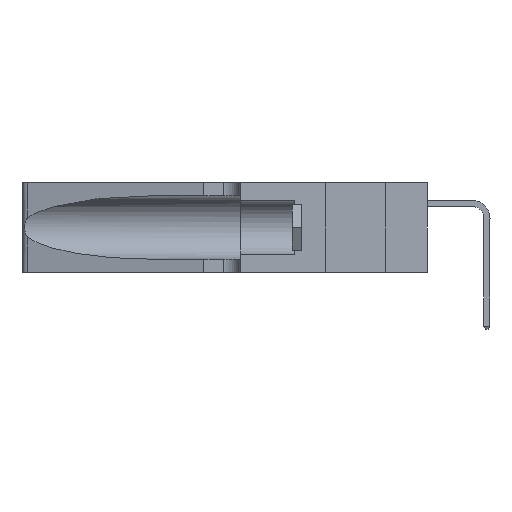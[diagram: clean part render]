
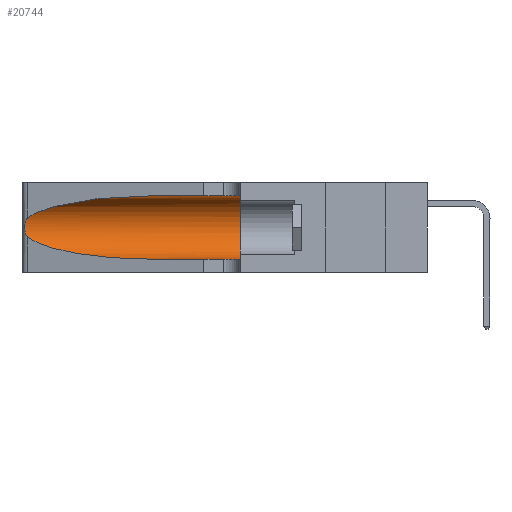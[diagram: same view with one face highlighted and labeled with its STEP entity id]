
A CAD part, left-side view. The second image highlights one B-rep face of the part: STEP entity #20744.
In plain terms, the highlighted cylindrical face has radius 3.308 mm (diameter 6.617 mm), a partial arc.
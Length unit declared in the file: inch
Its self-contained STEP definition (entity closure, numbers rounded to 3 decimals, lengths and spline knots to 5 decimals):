
#2457 = VERTEX_POINT ( 'NONE', #29035 ) ;
#2766 = CARTESIAN_POINT ( 'NONE',  ( 0.18966, 0.96281, 0.31525 ) ) ;
#2930 = CARTESIAN_POINT ( 'NONE',  ( 0.25555, 1.22993, 0.14849 ) ) ;
#2975 = DIRECTION ( 'NONE',  ( 0., 0., 1. ) ) ;
#4434 = CIRCLE ( 'NONE', #12523, 0.13025 ) ;
#4700 = VERTEX_POINT ( 'NONE', #17349 ) ;
#5155 = VERTEX_POINT ( 'NONE', #10146 ) ;
#5742 = VECTOR ( 'NONE', #9427, 39.37008 ) ;
#6196 = ORIENTED_EDGE ( 'NONE', *, *, #11854, .T. ) ;
#7155 = ORIENTED_EDGE ( 'NONE', *, *, #12592, .F. ) ;
#8852 = CARTESIAN_POINT ( 'NONE',  ( 0.25787, 1.23484, 0.2124 ) ) ;
#9427 = DIRECTION ( 'NONE',  ( 0., -1., 0. ) ) ;
#9533 =( BOUNDED_CURVE ( )  B_SPLINE_CURVE ( 3, ( #29793, #2766, #29912, #12100 ),
 .UNSPECIFIED., .F., .F. ) 
 B_SPLINE_CURVE_WITH_KNOTS ( ( 4, 4 ),
 ( 1.5708, 2.84003 ),
 .UNSPECIFIED. ) 
 CURVE ( )  GEOMETRIC_REPRESENTATION_ITEM ( )  RATIONAL_B_SPLINE_CURVE ( ( 1., 0.87, 0.87, 1. ) ) 
 REPRESENTATION_ITEM ( '' )  );
#10146 = CARTESIAN_POINT ( 'NONE',  ( 0.25487, 1.22718, 0.22369 ) ) ;
#10614 = CARTESIAN_POINT ( 'NONE',  ( 0.1305, 0.35, 0.185 ) ) ;
#10757 = ORIENTED_EDGE ( 'NONE', *, *, #21617, .T. ) ;
#11854 = EDGE_CURVE ( 'NONE', #20421, #36447, #29602, .T. ) ;
#11882 = CARTESIAN_POINT ( 'NONE',  ( 0.26018, 1.23835, 0.19895 ) ) ;
#12100 = CARTESIAN_POINT ( 'NONE',  ( 0.25487, 1.22718, 0.22369 ) ) ;
#12523 = AXIS2_PLACEMENT_3D ( 'NONE', #10614, #20919, #2975 ) ;
#12592 = EDGE_CURVE ( 'NONE', #4700, #2457, #34492, .T. ) ;
#13160 = B_SPLINE_CURVE_WITH_KNOTS ( 'NONE', 3,
 ( #38353, #32504, #26718, #8852, #29709, #11882, #32627, #14880, #35553, #17895, #38488, #20868, #2930, #23845 ),
 .UNSPECIFIED., .F., .F.,
 ( 4, 2, 2, 2, 2, 2, 4 ),
 ( 0., 0.00027, 0.00053, 0.00107, 0.0016, 0.00187, 0.00214 ),
 .UNSPECIFIED. ) ;
#14221 = CARTESIAN_POINT ( 'NONE',  ( 0.1305, 0.35, 0.05475 ) ) ;
#14829 = EDGE_CURVE ( 'NONE', #4700, #5155, #9533, .T. ) ;
#14880 = CARTESIAN_POINT ( 'NONE',  ( 0.26075, 1.23896, 0.178 ) ) ;
#15347 = EDGE_CURVE ( 'NONE', #2457, #36447, #4434, .T. ) ;
#15897 = CARTESIAN_POINT ( 'NONE',  ( 0.18966, 0.96281, 0.05475 ) ) ;
#16669 = VERTEX_POINT ( 'NONE', #26943 ) ;
#17170 = AXIS2_PLACEMENT_3D ( 'NONE', #28837, #25985, #20029 ) ;
#17349 = CARTESIAN_POINT ( 'NONE',  ( 0.1305, 0.72297, 0.31525 ) ) ;
#17895 = CARTESIAN_POINT ( 'NONE',  ( 0.25856, 1.23593, 0.16098 ) ) ;
#18598 = CYLINDRICAL_SURFACE ( 'NONE', #17170, 0.13025 ) ;
#18799 = CARTESIAN_POINT ( 'NONE',  ( 0.1305, 1.61858, 0.31525 ) ) ;
#19523 = FACE_OUTER_BOUND ( 'NONE', #21586, .T. ) ;
#20029 = DIRECTION ( 'NONE',  ( 0., 0., -1. ) ) ;
#20421 = VERTEX_POINT ( 'NONE', #33392 ) ;
#20744 = ADVANCED_FACE ( 'NONE', ( #19523 ), #18598, .F. ) ;
#20868 = CARTESIAN_POINT ( 'NONE',  ( 0.25639, 1.23186, 0.15144 ) ) ;
#20919 = DIRECTION ( 'NONE',  ( 0., 1., 0. ) ) ;
#21586 = EDGE_LOOP ( 'NONE', ( #27851, #10757, #31689, #6196, #37943, #7155 ) ) ;
#21617 = EDGE_CURVE ( 'NONE', #5155, #16669, #13160, .T. ) ;
#23845 = CARTESIAN_POINT ( 'NONE',  ( 0.25487, 1.22718, 0.14631 ) ) ;
#24277 = EDGE_CURVE ( 'NONE', #16669, #20421, #29727, .T. ) ;
#24756 = CARTESIAN_POINT ( 'NONE',  ( 0.2373, 1.15595, 0.08982 ) ) ;
#25985 = DIRECTION ( 'NONE',  ( 0., -1., 0. ) ) ;
#26718 = CARTESIAN_POINT ( 'NONE',  ( 0.25639, 1.23184, 0.21858 ) ) ;
#26729 = VECTOR ( 'NONE', #36441, 39.37008 ) ;
#26943 = CARTESIAN_POINT ( 'NONE',  ( 0.25487, 1.22718, 0.14631 ) ) ;
#27733 = CARTESIAN_POINT ( 'NONE',  ( 0.25487, 1.22718, 0.14631 ) ) ;
#27851 = ORIENTED_EDGE ( 'NONE', *, *, #14829, .T. ) ;
#28837 = CARTESIAN_POINT ( 'NONE',  ( 0.1305, 1.61858, 0.185 ) ) ;
#29035 = CARTESIAN_POINT ( 'NONE',  ( 0.1305, 0.35, 0.31525 ) ) ;
#29602 = LINE ( 'NONE', #30263, #5742 ) ;
#29709 = CARTESIAN_POINT ( 'NONE',  ( 0.25854, 1.2359, 0.20912 ) ) ;
#29727 =( BOUNDED_CURVE ( )  B_SPLINE_CURVE ( 3, ( #27733, #24756, #15897, #36566 ),
 .UNSPECIFIED., .F., .F. ) 
 B_SPLINE_CURVE_WITH_KNOTS ( ( 4, 4 ),
 ( 3.44316, 4.71239 ),
 .UNSPECIFIED. ) 
 CURVE ( )  GEOMETRIC_REPRESENTATION_ITEM ( )  RATIONAL_B_SPLINE_CURVE ( ( 1., 0.87, 0.87, 1. ) ) 
 REPRESENTATION_ITEM ( '' )  );
#29793 = CARTESIAN_POINT ( 'NONE',  ( 0.1305, 0.72297, 0.31525 ) ) ;
#29912 = CARTESIAN_POINT ( 'NONE',  ( 0.2373, 1.15595, 0.28018 ) ) ;
#30263 = CARTESIAN_POINT ( 'NONE',  ( 0.1305, 1.61858, 0.05475 ) ) ;
#31689 = ORIENTED_EDGE ( 'NONE', *, *, #24277, .T. ) ;
#32504 = CARTESIAN_POINT ( 'NONE',  ( 0.25555, 1.22994, 0.2215 ) ) ;
#32627 = CARTESIAN_POINT ( 'NONE',  ( 0.26075, 1.23896, 0.19203 ) ) ;
#33392 = CARTESIAN_POINT ( 'NONE',  ( 0.1305, 0.72297, 0.05475 ) ) ;
#34492 = LINE ( 'NONE', #18799, #26729 ) ;
#35553 = CARTESIAN_POINT ( 'NONE',  ( 0.26017, 1.23833, 0.17102 ) ) ;
#36441 = DIRECTION ( 'NONE',  ( 0., -1., 0. ) ) ;
#36447 = VERTEX_POINT ( 'NONE', #14221 ) ;
#36566 = CARTESIAN_POINT ( 'NONE',  ( 0.1305, 0.72297, 0.05475 ) ) ;
#37943 = ORIENTED_EDGE ( 'NONE', *, *, #15347, .F. ) ;
#38353 = CARTESIAN_POINT ( 'NONE',  ( 0.25487, 1.22718, 0.22369 ) ) ;
#38488 = CARTESIAN_POINT ( 'NONE',  ( 0.25789, 1.23486, 0.15765 ) ) ;
